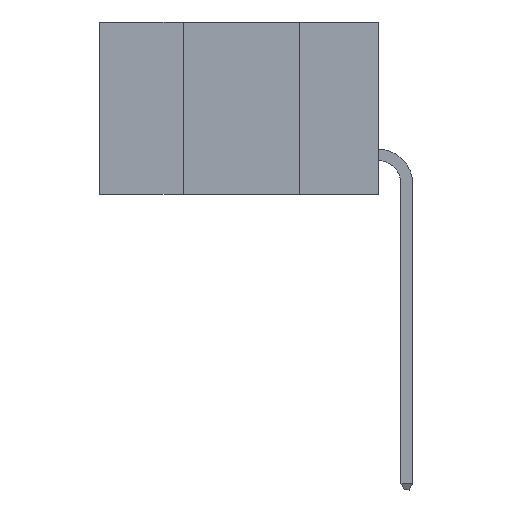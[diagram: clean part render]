
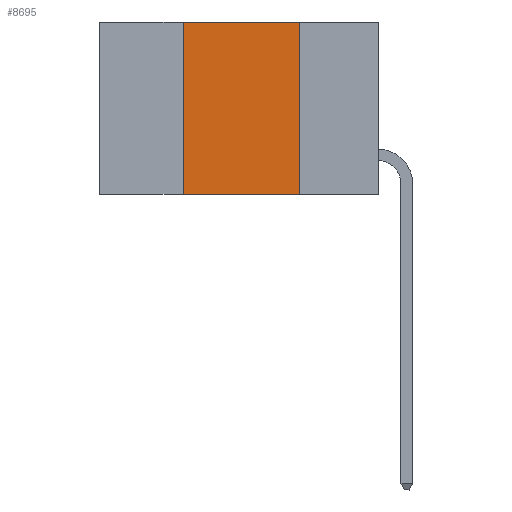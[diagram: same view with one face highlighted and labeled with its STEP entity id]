
A CAD part, left-side view. The second image highlights one B-rep face of the part: STEP entity #8695.
In plain terms, the highlighted planar face has unit normal (-1, 0, 0).
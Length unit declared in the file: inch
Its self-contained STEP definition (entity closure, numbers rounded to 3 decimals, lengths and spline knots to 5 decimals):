
#84 = CARTESIAN_POINT ( 'NONE',  ( 0., 0.6, 0. ) ) ;
#120 = DIRECTION ( 'NONE',  ( 0., 0., -1. ) ) ;
#811 = ORIENTED_EDGE ( 'NONE', *, *, #6286, .T. ) ;
#892 = VERTEX_POINT ( 'NONE', #7479 ) ;
#1229 = EDGE_CURVE ( 'NONE', #10012, #3740, #10277, .T. ) ;
#1335 = EDGE_CURVE ( 'NONE', #3740, #7155, #7987, .T. ) ;
#1795 = ORIENTED_EDGE ( 'NONE', *, *, #1229, .F. ) ;
#1922 = LINE ( 'NONE', #7530, #7554 ) ;
#2280 = FACE_OUTER_BOUND ( 'NONE', #4049, .T. ) ;
#2281 = DIRECTION ( 'NONE',  ( 0., 0., 1. ) ) ;
#2307 = CARTESIAN_POINT ( 'NONE',  ( 0., 0.6, -0.37 ) ) ;
#2449 = ORIENTED_EDGE ( 'NONE', *, *, #3495, .F. ) ;
#2873 = CARTESIAN_POINT ( 'NONE',  ( 0., 0.42, -0.37 ) ) ;
#3001 = LINE ( 'NONE', #2307, #5946 ) ;
#3148 = DIRECTION ( 'NONE',  ( 0., -1., 0. ) ) ;
#3489 = VECTOR ( 'NONE', #2281, 39.37008 ) ;
#3495 = EDGE_CURVE ( 'NONE', #7155, #892, #1922, .T. ) ;
#3740 = VERTEX_POINT ( 'NONE', #7473 ) ;
#4049 = EDGE_LOOP ( 'NONE', ( #2449, #10443, #1795, #811 ) ) ;
#4433 = AXIS2_PLACEMENT_3D ( 'NONE', #84, #8291, #120 ) ;
#4768 = CARTESIAN_POINT ( 'NONE',  ( 0., 0.42, 0. ) ) ;
#5107 = DIRECTION ( 'NONE',  ( 0., 0., -1. ) ) ;
#5277 = CARTESIAN_POINT ( 'NONE',  ( 0., 0.17, 0. ) ) ;
#5836 = DIRECTION ( 'NONE',  ( 0., -1., 0. ) ) ;
#5946 = VECTOR ( 'NONE', #3148, 39.37008 ) ;
#6286 = EDGE_CURVE ( 'NONE', #10012, #892, #3001, .T. ) ;
#6732 = CARTESIAN_POINT ( 'NONE',  ( 0., 0.6, 0. ) ) ;
#7155 = VERTEX_POINT ( 'NONE', #5277 ) ;
#7455 = PLANE ( 'NONE',  #4433 ) ;
#7473 = CARTESIAN_POINT ( 'NONE',  ( 0., 0.42, 0. ) ) ;
#7479 = CARTESIAN_POINT ( 'NONE',  ( 0., 0.17, -0.37 ) ) ;
#7530 = CARTESIAN_POINT ( 'NONE',  ( 0., 0.17, 0. ) ) ;
#7554 = VECTOR ( 'NONE', #5107, 39.37008 ) ;
#7987 = LINE ( 'NONE', #6732, #8993 ) ;
#8291 = DIRECTION ( 'NONE',  ( 1., 0., 0. ) ) ;
#8695 = ADVANCED_FACE ( 'NONE', ( #2280 ), #7455, .F. ) ;
#8993 = VECTOR ( 'NONE', #5836, 39.37008 ) ;
#10012 = VERTEX_POINT ( 'NONE', #2873 ) ;
#10277 = LINE ( 'NONE', #4768, #3489 ) ;
#10443 = ORIENTED_EDGE ( 'NONE', *, *, #1335, .F. ) ;
